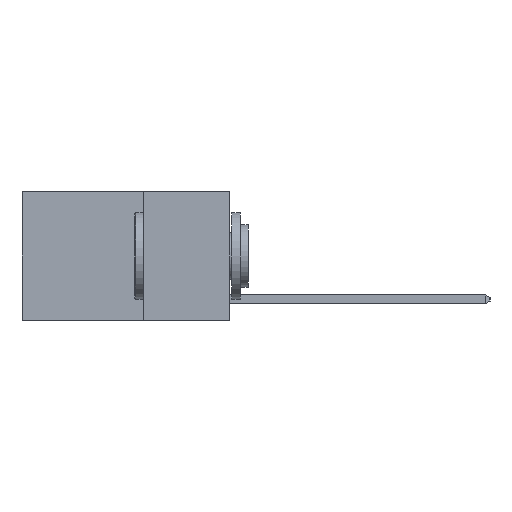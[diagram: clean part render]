
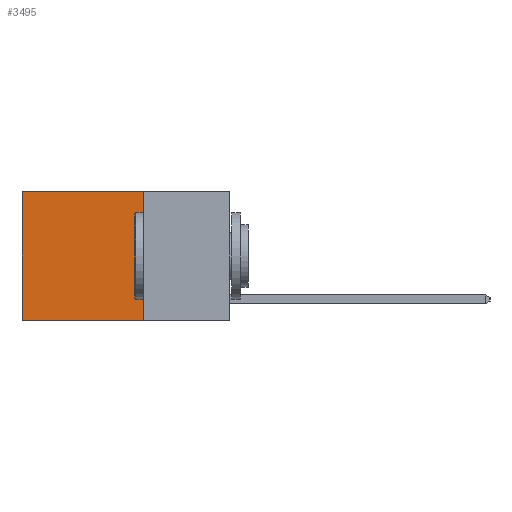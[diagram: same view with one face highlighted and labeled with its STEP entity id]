
A CAD part, left-side view. The second image highlights one B-rep face of the part: STEP entity #3495.
In plain terms, the highlighted planar face has unit normal (-1, 0, 0).
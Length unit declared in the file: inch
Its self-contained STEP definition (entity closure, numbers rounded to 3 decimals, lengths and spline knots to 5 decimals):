
#259 = CARTESIAN_POINT ( 'NONE',  ( 0.2625, 0.25, 0. ) ) ;
#1316 = ORIENTED_EDGE ( 'NONE', *, *, #9591, .T. ) ;
#1438 = CARTESIAN_POINT ( 'NONE',  ( 0.2625, 0.6, -0.37 ) ) ;
#1587 = EDGE_CURVE ( 'NONE', #2812, #7714, #10358, .T. ) ;
#1772 = CARTESIAN_POINT ( 'NONE',  ( 0.2625, 0.25, 0. ) ) ;
#2138 = LINE ( 'NONE', #1772, #9174 ) ;
#2362 = EDGE_LOOP ( 'NONE', ( #10422, #8382, #10692, #1316 ) ) ;
#2812 = VERTEX_POINT ( 'NONE', #259 ) ;
#3495 = ADVANCED_FACE ( 'NONE', ( #4766 ), #9132, .F. ) ;
#3558 = EDGE_CURVE ( 'NONE', #4890, #8411, #7998, .T. ) ;
#4123 = VECTOR ( 'NONE', #6210, 39.37008 ) ;
#4766 = FACE_OUTER_BOUND ( 'NONE', #2362, .T. ) ;
#4823 = DIRECTION ( 'NONE',  ( 1., 0., 0. ) ) ;
#4890 = VERTEX_POINT ( 'NONE', #11267 ) ;
#5956 = CARTESIAN_POINT ( 'NONE',  ( 0.2625, 0.6, 0. ) ) ;
#6210 = DIRECTION ( 'NONE',  ( 0., 1., 0. ) ) ;
#6310 = DIRECTION ( 'NONE',  ( 0., 0., -1. ) ) ;
#6629 = LINE ( 'NONE', #7848, #4123 ) ;
#6902 = AXIS2_PLACEMENT_3D ( 'NONE', #8235, #4823, #10854 ) ;
#7714 = VERTEX_POINT ( 'NONE', #11553 ) ;
#7781 = VECTOR ( 'NONE', #6310, 39.37008 ) ;
#7848 = CARTESIAN_POINT ( 'NONE',  ( 0.2625, 0.25, -0.37 ) ) ;
#7998 = LINE ( 'NONE', #5956, #10329 ) ;
#8235 = CARTESIAN_POINT ( 'NONE',  ( 0.2625, 0.25, 0. ) ) ;
#8382 = ORIENTED_EDGE ( 'NONE', *, *, #10897, .F. ) ;
#8411 = VERTEX_POINT ( 'NONE', #1438 ) ;
#9132 = PLANE ( 'NONE',  #6902 ) ;
#9174 = VECTOR ( 'NONE', #10806, 39.37008 ) ;
#9591 = EDGE_CURVE ( 'NONE', #2812, #4890, #2138, .T. ) ;
#10055 = CARTESIAN_POINT ( 'NONE',  ( 0.2625, 0.25, 0. ) ) ;
#10329 = VECTOR ( 'NONE', #10990, 39.37008 ) ;
#10358 = LINE ( 'NONE', #10055, #7781 ) ;
#10422 = ORIENTED_EDGE ( 'NONE', *, *, #3558, .T. ) ;
#10692 = ORIENTED_EDGE ( 'NONE', *, *, #1587, .F. ) ;
#10806 = DIRECTION ( 'NONE',  ( 0., 1., 0. ) ) ;
#10854 = DIRECTION ( 'NONE',  ( 0., 0., -1. ) ) ;
#10897 = EDGE_CURVE ( 'NONE', #7714, #8411, #6629, .T. ) ;
#10990 = DIRECTION ( 'NONE',  ( 0., 0., -1. ) ) ;
#11267 = CARTESIAN_POINT ( 'NONE',  ( 0.2625, 0.6, 0. ) ) ;
#11553 = CARTESIAN_POINT ( 'NONE',  ( 0.2625, 0.25, -0.37 ) ) ;
